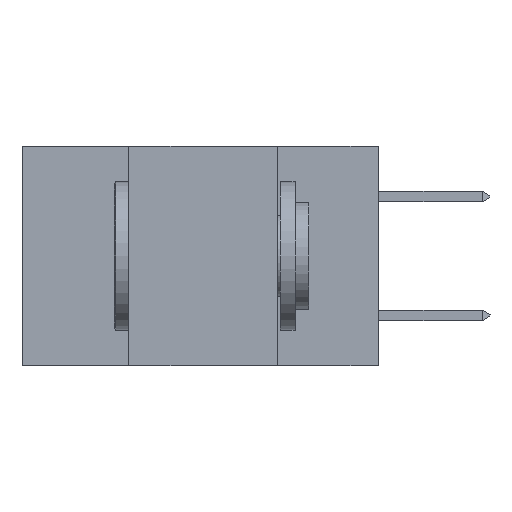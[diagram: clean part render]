
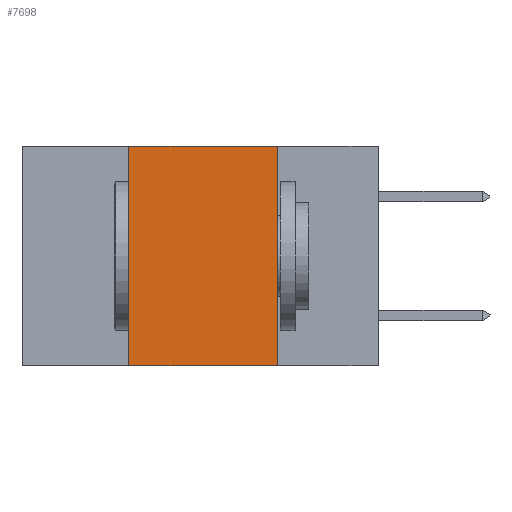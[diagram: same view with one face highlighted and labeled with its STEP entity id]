
A CAD part, left-side view. The second image highlights one B-rep face of the part: STEP entity #7698.
In plain terms, the highlighted planar face has unit normal (-1, 0, 0).
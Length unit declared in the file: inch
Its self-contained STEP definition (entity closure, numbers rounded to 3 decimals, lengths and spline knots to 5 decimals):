
#631 = ORIENTED_EDGE ( 'NONE', *, *, #3381, .F. ) ;
#660 = CARTESIAN_POINT ( 'NONE',  ( 0., 0.17, 0. ) ) ;
#1080 = DIRECTION ( 'NONE',  ( 0., 0., 1. ) ) ;
#2006 = CARTESIAN_POINT ( 'NONE',  ( 0., 0.6, -0.37 ) ) ;
#2038 = ORIENTED_EDGE ( 'NONE', *, *, #17899, .T. ) ;
#2469 = CARTESIAN_POINT ( 'NONE',  ( 0., 0.6, 0. ) ) ;
#2862 = EDGE_LOOP ( 'NONE', ( #12599, #631, #6077, #2038 ) ) ;
#3381 = EDGE_CURVE ( 'NONE', #6001, #9757, #17227, .T. ) ;
#3942 = VECTOR ( 'NONE', #8236, 39.37008 ) ;
#5823 = CARTESIAN_POINT ( 'NONE',  ( 0., 0.42, 0. ) ) ;
#6001 = VERTEX_POINT ( 'NONE', #13753 ) ;
#6077 = ORIENTED_EDGE ( 'NONE', *, *, #8441, .F. ) ;
#6399 = LINE ( 'NONE', #2006, #3942 ) ;
#7698 = ADVANCED_FACE ( 'NONE', ( #16322 ), #18575, .F. ) ;
#8236 = DIRECTION ( 'NONE',  ( 0., -1., 0. ) ) ;
#8441 = EDGE_CURVE ( 'NONE', #15024, #6001, #11335, .T. ) ;
#9618 = VECTOR ( 'NONE', #1080, 39.37008 ) ;
#9757 = VERTEX_POINT ( 'NONE', #660 ) ;
#10276 = DIRECTION ( 'NONE',  ( 0., 0., -1. ) ) ;
#10347 = CARTESIAN_POINT ( 'NONE',  ( 0., 0.17, 0. ) ) ;
#10866 = AXIS2_PLACEMENT_3D ( 'NONE', #2469, #13744, #13541 ) ;
#11335 = LINE ( 'NONE', #5823, #9618 ) ;
#11514 = CARTESIAN_POINT ( 'NONE',  ( 0., 0.42, -0.37 ) ) ;
#11563 = VECTOR ( 'NONE', #10276, 39.37008 ) ;
#12599 = ORIENTED_EDGE ( 'NONE', *, *, #18756, .F. ) ;
#12840 = DIRECTION ( 'NONE',  ( 0., -1., 0. ) ) ;
#12940 = VERTEX_POINT ( 'NONE', #17943 ) ;
#13541 = DIRECTION ( 'NONE',  ( 0., 0., -1. ) ) ;
#13744 = DIRECTION ( 'NONE',  ( 1., 0., 0. ) ) ;
#13753 = CARTESIAN_POINT ( 'NONE',  ( 0., 0.42, 0. ) ) ;
#15024 = VERTEX_POINT ( 'NONE', #11514 ) ;
#15764 = LINE ( 'NONE', #10347, #11563 ) ;
#16228 = CARTESIAN_POINT ( 'NONE',  ( 0., 0.6, 0. ) ) ;
#16322 = FACE_OUTER_BOUND ( 'NONE', #2862, .T. ) ;
#17004 = VECTOR ( 'NONE', #12840, 39.37008 ) ;
#17227 = LINE ( 'NONE', #16228, #17004 ) ;
#17899 = EDGE_CURVE ( 'NONE', #15024, #12940, #6399, .T. ) ;
#17943 = CARTESIAN_POINT ( 'NONE',  ( 0., 0.17, -0.37 ) ) ;
#18575 = PLANE ( 'NONE',  #10866 ) ;
#18756 = EDGE_CURVE ( 'NONE', #9757, #12940, #15764, .T. ) ;
